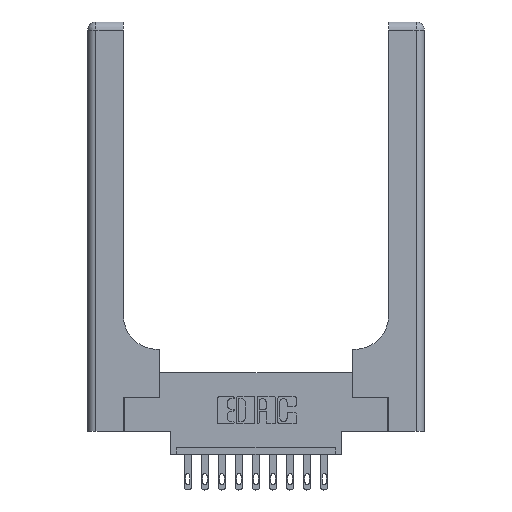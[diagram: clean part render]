
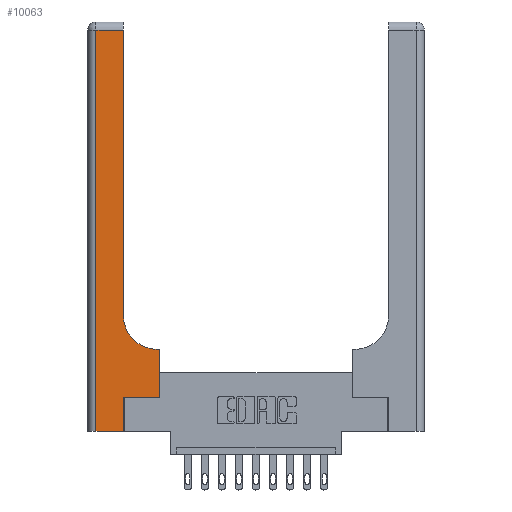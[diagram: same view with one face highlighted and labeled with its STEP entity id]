
A CAD part, top view. The second image highlights one B-rep face of the part: STEP entity #10063.
In plain terms, the highlighted planar face has unit normal (0, 0, 1).
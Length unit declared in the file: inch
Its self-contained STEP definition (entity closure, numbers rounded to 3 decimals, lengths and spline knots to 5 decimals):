
#739 = ORIENTED_EDGE ( 'NONE', *, *, #8576, .T. ) ;
#807 = LINE ( 'NONE', #9384, #2195 ) ;
#906 = CIRCLE ( 'NONE', #7257, 0.25 ) ;
#1049 = VERTEX_POINT ( 'NONE', #4711 ) ;
#1061 = DIRECTION ( 'NONE',  ( 0., 1., 0. ) ) ;
#1254 = VERTEX_POINT ( 'NONE', #13392 ) ;
#1290 = DIRECTION ( 'NONE',  ( -1., 0., 0. ) ) ;
#2151 = VECTOR ( 'NONE', #7157, 39.37008 ) ;
#2195 = VECTOR ( 'NONE', #11933, 39.37008 ) ;
#2466 = CARTESIAN_POINT ( 'NONE',  ( 0.265, 0.25, 0.37 ) ) ;
#2702 = DIRECTION ( 'NONE',  ( -1., 0., 0. ) ) ;
#3098 = EDGE_CURVE ( 'NONE', #4994, #7835, #5639, .T. ) ;
#3171 = VECTOR ( 'NONE', #1061, 39.37008 ) ;
#3414 = PLANE ( 'NONE',  #6234 ) ;
#3973 = LINE ( 'NONE', #6295, #13353 ) ;
#4125 = VERTEX_POINT ( 'NONE', #12826 ) ;
#4305 = CARTESIAN_POINT ( 'NONE',  ( 0.06, 0., 0.37 ) ) ;
#4623 = ORIENTED_EDGE ( 'NONE', *, *, #13669, .T. ) ;
#4691 = VECTOR ( 'NONE', #10949, 39.37008 ) ;
#4711 = CARTESIAN_POINT ( 'NONE',  ( 0.528, 0.25, 0.37 ) ) ;
#4786 = VECTOR ( 'NONE', #7319, 39.37008 ) ;
#4994 = VERTEX_POINT ( 'NONE', #13117 ) ;
#5639 = LINE ( 'NONE', #9286, #13360 ) ;
#6041 = LINE ( 'NONE', #8339, #2151 ) ;
#6135 = LINE ( 'NONE', #9620, #4786 ) ;
#6234 = AXIS2_PLACEMENT_3D ( 'NONE', #9711, #14635, #1290 ) ;
#6295 = CARTESIAN_POINT ( 'NONE',  ( 0., 2.94, 0.37 ) ) ;
#7005 = ORIENTED_EDGE ( 'NONE', *, *, #12394, .T. ) ;
#7006 = LINE ( 'NONE', #10903, #11714 ) ;
#7114 = LINE ( 'NONE', #8620, #3171 ) ;
#7157 = DIRECTION ( 'NONE',  ( 0., -1., 0. ) ) ;
#7185 = CARTESIAN_POINT ( 'NONE',  ( 0.51, 0.85, 0.37 ) ) ;
#7257 = AXIS2_PLACEMENT_3D ( 'NONE', #7185, #12031, #15686 ) ;
#7319 = DIRECTION ( 'NONE',  ( 1., 0., 0. ) ) ;
#7389 = ORIENTED_EDGE ( 'NONE', *, *, #10426, .T. ) ;
#7453 = ORIENTED_EDGE ( 'NONE', *, *, #7721, .T. ) ;
#7721 = EDGE_CURVE ( 'NONE', #11812, #8284, #7006, .T. ) ;
#7835 = VERTEX_POINT ( 'NONE', #2466 ) ;
#8284 = VERTEX_POINT ( 'NONE', #14255 ) ;
#8339 = CARTESIAN_POINT ( 'NONE',  ( 0.06, 3., 0.37 ) ) ;
#8576 = EDGE_CURVE ( 'NONE', #1049, #11812, #7114, .T. ) ;
#8588 = EDGE_CURVE ( 'NONE', #8284, #13548, #906, .T. ) ;
#8620 = CARTESIAN_POINT ( 'NONE',  ( 0.528, 0.25, 0.37 ) ) ;
#9220 = CARTESIAN_POINT ( 'NONE',  ( 0.26, 0.85, 0.37 ) ) ;
#9286 = CARTESIAN_POINT ( 'NONE',  ( 0.265, 0., 0.37 ) ) ;
#9384 = CARTESIAN_POINT ( 'NONE',  ( 0.265, 0.25, 0.37 ) ) ;
#9620 = CARTESIAN_POINT ( 'NONE',  ( 0., 0., 0.37 ) ) ;
#9711 = CARTESIAN_POINT ( 'NONE',  ( 0., 3., 0.37 ) ) ;
#9736 = EDGE_LOOP ( 'NONE', ( #12915, #10257, #7389, #4623, #10098, #7005, #739, #7453, #11419 ) ) ;
#9869 = EDGE_CURVE ( 'NONE', #13548, #4125, #14820, .T. ) ;
#10063 = ADVANCED_FACE ( 'NONE', ( #10664 ), #3414, .F. ) ;
#10098 = ORIENTED_EDGE ( 'NONE', *, *, #3098, .T. ) ;
#10235 = EDGE_CURVE ( 'NONE', #4125, #1254, #3973, .T. ) ;
#10257 = ORIENTED_EDGE ( 'NONE', *, *, #10235, .T. ) ;
#10406 = DIRECTION ( 'NONE',  ( 0., 1., 0. ) ) ;
#10426 = EDGE_CURVE ( 'NONE', #1254, #11878, #6041, .T. ) ;
#10664 = FACE_OUTER_BOUND ( 'NONE', #9736, .T. ) ;
#10903 = CARTESIAN_POINT ( 'NONE',  ( 0.26, 0.6, 0.37 ) ) ;
#10949 = DIRECTION ( 'NONE',  ( 0., 1., 0. ) ) ;
#11265 = CARTESIAN_POINT ( 'NONE',  ( 0.26, 3., 0.37 ) ) ;
#11419 = ORIENTED_EDGE ( 'NONE', *, *, #8588, .T. ) ;
#11714 = VECTOR ( 'NONE', #15665, 39.37008 ) ;
#11812 = VERTEX_POINT ( 'NONE', #13479 ) ;
#11878 = VERTEX_POINT ( 'NONE', #4305 ) ;
#11933 = DIRECTION ( 'NONE',  ( 1., 0., 0. ) ) ;
#12031 = DIRECTION ( 'NONE',  ( 0., 0., -1. ) ) ;
#12394 = EDGE_CURVE ( 'NONE', #7835, #1049, #807, .T. ) ;
#12826 = CARTESIAN_POINT ( 'NONE',  ( 0.26, 2.94, 0.37 ) ) ;
#12915 = ORIENTED_EDGE ( 'NONE', *, *, #9869, .T. ) ;
#13117 = CARTESIAN_POINT ( 'NONE',  ( 0.265, 0., 0.37 ) ) ;
#13353 = VECTOR ( 'NONE', #2702, 39.37008 ) ;
#13360 = VECTOR ( 'NONE', #10406, 39.37008 ) ;
#13392 = CARTESIAN_POINT ( 'NONE',  ( 0.06, 2.94, 0.37 ) ) ;
#13479 = CARTESIAN_POINT ( 'NONE',  ( 0.528, 0.6, 0.37 ) ) ;
#13548 = VERTEX_POINT ( 'NONE', #9220 ) ;
#13669 = EDGE_CURVE ( 'NONE', #11878, #4994, #6135, .T. ) ;
#14255 = CARTESIAN_POINT ( 'NONE',  ( 0.51, 0.6, 0.37 ) ) ;
#14635 = DIRECTION ( 'NONE',  ( 0., 0., -1. ) ) ;
#14820 = LINE ( 'NONE', #11265, #4691 ) ;
#15665 = DIRECTION ( 'NONE',  ( -1., 0., 0. ) ) ;
#15686 = DIRECTION ( 'NONE',  ( 1., 0., 0. ) ) ;
